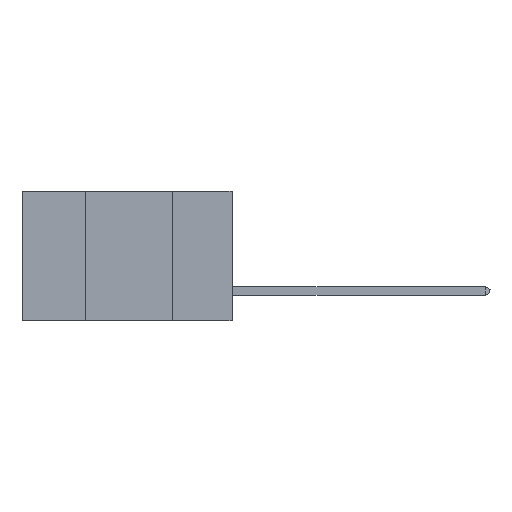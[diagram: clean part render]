
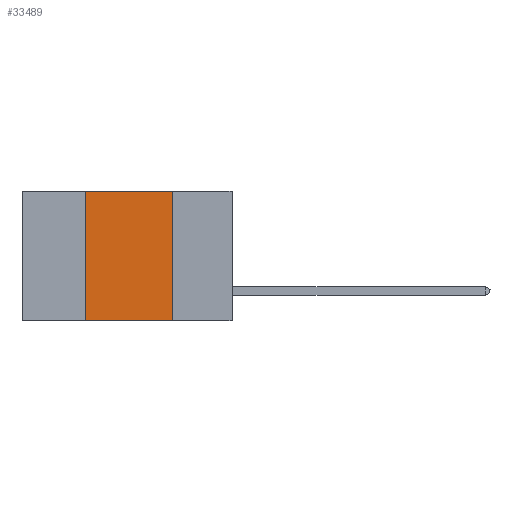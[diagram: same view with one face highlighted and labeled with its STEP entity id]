
A CAD part, left-side view. The second image highlights one B-rep face of the part: STEP entity #33489.
In plain terms, the highlighted planar face has unit normal (-1, 0, 0).
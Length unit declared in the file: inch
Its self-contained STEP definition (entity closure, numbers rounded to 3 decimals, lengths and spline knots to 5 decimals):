
#1313 = VECTOR ( 'NONE', #26900, 39.37008 ) ;
#1794 = ORIENTED_EDGE ( 'NONE', *, *, #11389, .F. ) ;
#2124 = VERTEX_POINT ( 'NONE', #16400 ) ;
#2495 = CARTESIAN_POINT ( 'NONE',  ( 0., 0.6, 0. ) ) ;
#2831 = DIRECTION ( 'NONE',  ( 0., 0., -1. ) ) ;
#3089 = CARTESIAN_POINT ( 'NONE',  ( 0., 0.6, 0. ) ) ;
#3859 = VECTOR ( 'NONE', #16691, 39.37008 ) ;
#5187 = DIRECTION ( 'NONE',  ( 1., 0., 0. ) ) ;
#6187 = VERTEX_POINT ( 'NONE', #12204 ) ;
#6908 = VERTEX_POINT ( 'NONE', #31181 ) ;
#11389 = EDGE_CURVE ( 'NONE', #2124, #6908, #28951, .T. ) ;
#12204 = CARTESIAN_POINT ( 'NONE',  ( 0., 0.42, -0.37 ) ) ;
#13076 = ORIENTED_EDGE ( 'NONE', *, *, #28688, .T. ) ;
#16287 = EDGE_CURVE ( 'NONE', #6187, #34436, #29919, .T. ) ;
#16400 = CARTESIAN_POINT ( 'NONE',  ( 0., 0.17, 0. ) ) ;
#16691 = DIRECTION ( 'NONE',  ( 0., -1., 0. ) ) ;
#17451 = CARTESIAN_POINT ( 'NONE',  ( 0., 0.17, 0. ) ) ;
#17975 = VECTOR ( 'NONE', #19806, 39.37008 ) ;
#18837 = ORIENTED_EDGE ( 'NONE', *, *, #16287, .F. ) ;
#19594 = VECTOR ( 'NONE', #31183, 39.37008 ) ;
#19806 = DIRECTION ( 'NONE',  ( 0., 0., -1. ) ) ;
#21325 = EDGE_LOOP ( 'NONE', ( #1794, #29147, #18837, #13076 ) ) ;
#21587 = CARTESIAN_POINT ( 'NONE',  ( 0., 0.42, 0. ) ) ;
#26395 = EDGE_CURVE ( 'NONE', #34436, #2124, #26972, .T. ) ;
#26900 = DIRECTION ( 'NONE',  ( 0., 0., 1. ) ) ;
#26972 = LINE ( 'NONE', #3089, #3859 ) ;
#28275 = AXIS2_PLACEMENT_3D ( 'NONE', #2495, #5187, #2831 ) ;
#28472 = LINE ( 'NONE', #28478, #19594 ) ;
#28478 = CARTESIAN_POINT ( 'NONE',  ( 0., 0.6, -0.37 ) ) ;
#28509 = CARTESIAN_POINT ( 'NONE',  ( 0., 0.42, 0. ) ) ;
#28688 = EDGE_CURVE ( 'NONE', #6187, #6908, #28472, .T. ) ;
#28951 = LINE ( 'NONE', #17451, #17975 ) ;
#29147 = ORIENTED_EDGE ( 'NONE', *, *, #26395, .F. ) ;
#29919 = LINE ( 'NONE', #21587, #1313 ) ;
#31181 = CARTESIAN_POINT ( 'NONE',  ( 0., 0.17, -0.37 ) ) ;
#31183 = DIRECTION ( 'NONE',  ( 0., -1., 0. ) ) ;
#31953 = FACE_OUTER_BOUND ( 'NONE', #21325, .T. ) ;
#33489 = ADVANCED_FACE ( 'NONE', ( #31953 ), #34670, .F. ) ;
#34436 = VERTEX_POINT ( 'NONE', #28509 ) ;
#34670 = PLANE ( 'NONE',  #28275 ) ;
